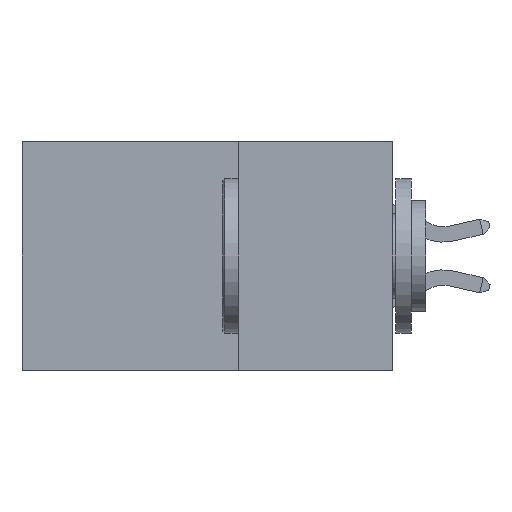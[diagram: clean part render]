
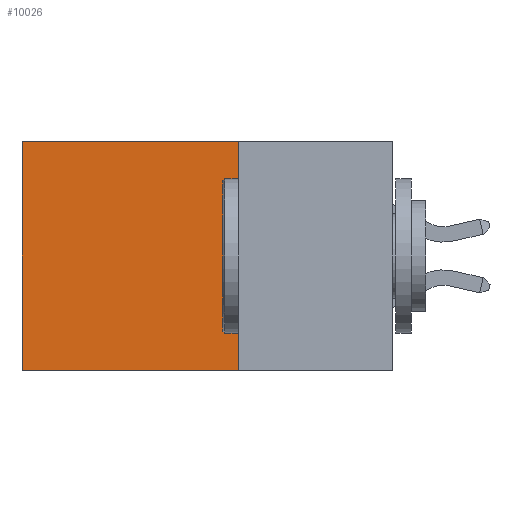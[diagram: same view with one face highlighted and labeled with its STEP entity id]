
A CAD part, left-side view. The second image highlights one B-rep face of the part: STEP entity #10026.
In plain terms, the highlighted planar face has unit normal (-1, 0, 0).
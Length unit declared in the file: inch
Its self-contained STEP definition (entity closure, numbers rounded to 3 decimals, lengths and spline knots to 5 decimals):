
#993 = DIRECTION ( 'NONE',  ( 0., 0., -1. ) ) ;
#2193 = DIRECTION ( 'NONE',  ( 0., 0., -1. ) ) ;
#2314 = VERTEX_POINT ( 'NONE', #6993 ) ;
#2869 = VECTOR ( 'NONE', #23552, 39.37008 ) ;
#3640 = CARTESIAN_POINT ( 'NONE',  ( 0.2875, 0.6, 0. ) ) ;
#3798 = CARTESIAN_POINT ( 'NONE',  ( 0.2875, 0.6, 0. ) ) ;
#5772 = ORIENTED_EDGE ( 'NONE', *, *, #31000, .F. ) ;
#6095 = EDGE_CURVE ( 'NONE', #31328, #16213, #20432, .T. ) ;
#6729 = DIRECTION ( 'NONE',  ( 0., 0., -1. ) ) ;
#6993 = CARTESIAN_POINT ( 'NONE',  ( 0.2875, 0.25, 0. ) ) ;
#10026 = ADVANCED_FACE ( 'NONE', ( #25785 ), #19758, .F. ) ;
#11668 = ORIENTED_EDGE ( 'NONE', *, *, #6095, .F. ) ;
#11689 = EDGE_LOOP ( 'NONE', ( #28338, #11668, #5772, #18900 ) ) ;
#12082 = CARTESIAN_POINT ( 'NONE',  ( 0.2875, 0.25, 0. ) ) ;
#14674 = CARTESIAN_POINT ( 'NONE',  ( 0.2875, 0.25, 0. ) ) ;
#15088 = VERTEX_POINT ( 'NONE', #3640 ) ;
#16213 = VERTEX_POINT ( 'NONE', #27421 ) ;
#17221 = VECTOR ( 'NONE', #6729, 39.37008 ) ;
#17800 = DIRECTION ( 'NONE',  ( 0., 1., 0. ) ) ;
#18486 = AXIS2_PLACEMENT_3D ( 'NONE', #14674, #32578, #2193 ) ;
#18900 = ORIENTED_EDGE ( 'NONE', *, *, #31259, .T. ) ;
#19629 = VECTOR ( 'NONE', #17800, 39.37008 ) ;
#19758 = PLANE ( 'NONE',  #18486 ) ;
#20432 = LINE ( 'NONE', #26598, #19629 ) ;
#23444 = CARTESIAN_POINT ( 'NONE',  ( 0.2875, 0.25, 0. ) ) ;
#23552 = DIRECTION ( 'NONE',  ( 0., 1., 0. ) ) ;
#24048 = LINE ( 'NONE', #12082, #17221 ) ;
#25785 = FACE_OUTER_BOUND ( 'NONE', #11689, .T. ) ;
#26598 = CARTESIAN_POINT ( 'NONE',  ( 0.2875, 0.25, -0.37 ) ) ;
#27421 = CARTESIAN_POINT ( 'NONE',  ( 0.2875, 0.6, -0.37 ) ) ;
#27751 = EDGE_CURVE ( 'NONE', #15088, #16213, #29451, .T. ) ;
#28338 = ORIENTED_EDGE ( 'NONE', *, *, #27751, .T. ) ;
#28668 = VECTOR ( 'NONE', #993, 39.37008 ) ;
#29451 = LINE ( 'NONE', #3798, #28668 ) ;
#30132 = LINE ( 'NONE', #23444, #2869 ) ;
#31000 = EDGE_CURVE ( 'NONE', #2314, #31328, #24048, .T. ) ;
#31259 = EDGE_CURVE ( 'NONE', #2314, #15088, #30132, .T. ) ;
#31328 = VERTEX_POINT ( 'NONE', #31452 ) ;
#31452 = CARTESIAN_POINT ( 'NONE',  ( 0.2875, 0.25, -0.37 ) ) ;
#32578 = DIRECTION ( 'NONE',  ( 1., 0., 0. ) ) ;
